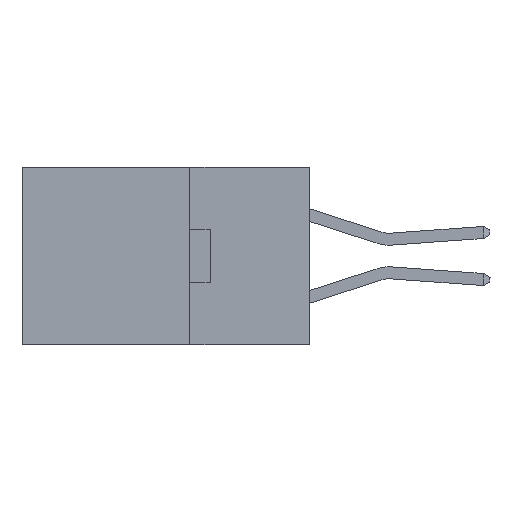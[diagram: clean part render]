
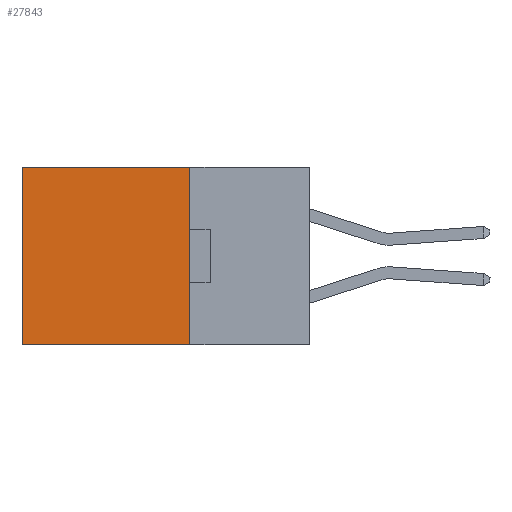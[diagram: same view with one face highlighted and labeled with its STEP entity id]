
A CAD part, left-side view. The second image highlights one B-rep face of the part: STEP entity #27843.
In plain terms, the highlighted planar face has unit normal (-1, 0, 0).
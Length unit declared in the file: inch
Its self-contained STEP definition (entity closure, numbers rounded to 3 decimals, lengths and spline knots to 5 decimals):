
#809 = VECTOR ( 'NONE', #5528, 39.37008 ) ;
#2359 = CARTESIAN_POINT ( 'NONE',  ( 0.2615, 0.25, -0.37 ) ) ;
#2910 = CARTESIAN_POINT ( 'NONE',  ( 0.2615, 0.6, 0. ) ) ;
#3080 = ORIENTED_EDGE ( 'NONE', *, *, #8252, .T. ) ;
#3405 = DIRECTION ( 'NONE',  ( 0., 0., -1. ) ) ;
#4707 = DIRECTION ( 'NONE',  ( 0., 0., -1. ) ) ;
#4738 = ORIENTED_EDGE ( 'NONE', *, *, #11463, .F. ) ;
#5495 = VERTEX_POINT ( 'NONE', #2910 ) ;
#5528 = DIRECTION ( 'NONE',  ( 0., 1., 0. ) ) ;
#7314 = VECTOR ( 'NONE', #11293, 39.37008 ) ;
#7780 = FACE_OUTER_BOUND ( 'NONE', #27477, .T. ) ;
#8252 = EDGE_CURVE ( 'NONE', #13613, #5495, #12797, .T. ) ;
#9595 = VECTOR ( 'NONE', #27110, 39.37008 ) ;
#9959 = CARTESIAN_POINT ( 'NONE',  ( 0.2615, 0.25, -0.37 ) ) ;
#10758 = VECTOR ( 'NONE', #3405, 39.37008 ) ;
#11293 = DIRECTION ( 'NONE',  ( 0., 0., -1. ) ) ;
#11463 = EDGE_CURVE ( 'NONE', #13613, #12771, #19239, .T. ) ;
#11980 = ORIENTED_EDGE ( 'NONE', *, *, #27137, .F. ) ;
#12771 = VERTEX_POINT ( 'NONE', #9959 ) ;
#12797 = LINE ( 'NONE', #25469, #809 ) ;
#13613 = VERTEX_POINT ( 'NONE', #15173 ) ;
#13937 = CARTESIAN_POINT ( 'NONE',  ( 0.2615, 0.25, -0.37 ) ) ;
#15145 = EDGE_CURVE ( 'NONE', #5495, #26605, #24651, .T. ) ;
#15173 = CARTESIAN_POINT ( 'NONE',  ( 0.2615, 0.25, 0. ) ) ;
#15981 = PLANE ( 'NONE',  #17647 ) ;
#16328 = ORIENTED_EDGE ( 'NONE', *, *, #15145, .T. ) ;
#17003 = LINE ( 'NONE', #13937, #9595 ) ;
#17647 = AXIS2_PLACEMENT_3D ( 'NONE', #2359, #18196, #4707 ) ;
#18196 = DIRECTION ( 'NONE',  ( 1., 0., 0. ) ) ;
#19239 = LINE ( 'NONE', #20178, #7314 ) ;
#20178 = CARTESIAN_POINT ( 'NONE',  ( 0.2615, 0.25, -0.37 ) ) ;
#21330 = CARTESIAN_POINT ( 'NONE',  ( 0.2615, 0.6, -0.37 ) ) ;
#24651 = LINE ( 'NONE', #21330, #10758 ) ;
#25469 = CARTESIAN_POINT ( 'NONE',  ( 0.2615, 0.25, 0. ) ) ;
#25488 = CARTESIAN_POINT ( 'NONE',  ( 0.2615, 0.6, -0.37 ) ) ;
#26605 = VERTEX_POINT ( 'NONE', #25488 ) ;
#27110 = DIRECTION ( 'NONE',  ( 0., 1., 0. ) ) ;
#27137 = EDGE_CURVE ( 'NONE', #12771, #26605, #17003, .T. ) ;
#27477 = EDGE_LOOP ( 'NONE', ( #16328, #11980, #4738, #3080 ) ) ;
#27843 = ADVANCED_FACE ( 'NONE', ( #7780 ), #15981, .F. ) ;
